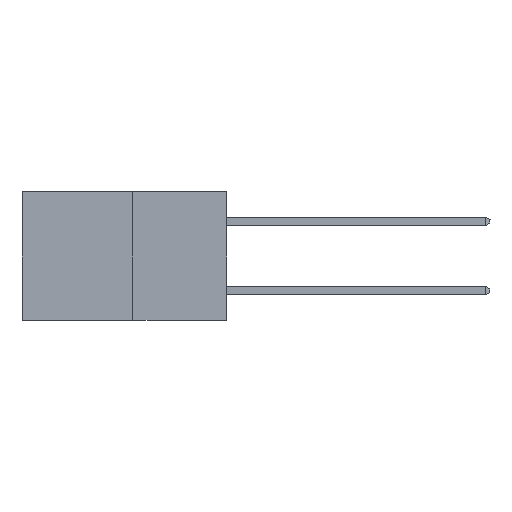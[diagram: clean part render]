
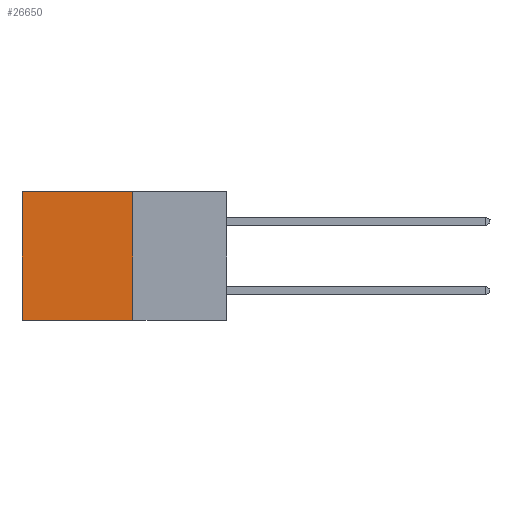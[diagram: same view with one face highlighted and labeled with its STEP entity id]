
A CAD part, left-side view. The second image highlights one B-rep face of the part: STEP entity #26650.
In plain terms, the highlighted planar face has unit normal (-1, 0, 0).
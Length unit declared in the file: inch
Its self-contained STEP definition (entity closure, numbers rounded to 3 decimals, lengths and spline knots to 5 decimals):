
#1404 = CARTESIAN_POINT ( 'NONE',  ( 0.277, 0.27, -0.37 ) ) ;
#2034 = LINE ( 'NONE', #11757, #30102 ) ;
#2102 = LINE ( 'NONE', #32947, #27060 ) ;
#2589 = CARTESIAN_POINT ( 'NONE',  ( 0.277, 0.59, 0. ) ) ;
#3235 = VERTEX_POINT ( 'NONE', #30724 ) ;
#3621 = CARTESIAN_POINT ( 'NONE',  ( 0.277, 0.59, -0.37 ) ) ;
#4065 = DIRECTION ( 'NONE',  ( 1., 0., 0. ) ) ;
#5108 = EDGE_CURVE ( 'NONE', #29380, #3235, #18339, .T. ) ;
#5743 = CARTESIAN_POINT ( 'NONE',  ( 0.277, 0.27, -0.37 ) ) ;
#5792 = DIRECTION ( 'NONE',  ( 0., 0., -1. ) ) ;
#6982 = EDGE_CURVE ( 'NONE', #18770, #32839, #2034, .T. ) ;
#7533 = VECTOR ( 'NONE', #29878, 39.37008 ) ;
#7955 = EDGE_LOOP ( 'NONE', ( #28586, #11319, #18365, #10994 ) ) ;
#9662 = DIRECTION ( 'NONE',  ( 0., 0., -1. ) ) ;
#10994 = ORIENTED_EDGE ( 'NONE', *, *, #12535, .T. ) ;
#11319 = ORIENTED_EDGE ( 'NONE', *, *, #11632, .F. ) ;
#11632 = EDGE_CURVE ( 'NONE', #3235, #32839, #21227, .T. ) ;
#11757 = CARTESIAN_POINT ( 'NONE',  ( 0.277, 0.59, -0.37 ) ) ;
#12535 = EDGE_CURVE ( 'NONE', #29380, #18770, #2102, .T. ) ;
#13899 = FACE_OUTER_BOUND ( 'NONE', #7955, .T. ) ;
#15368 = AXIS2_PLACEMENT_3D ( 'NONE', #1404, #4065, #22127 ) ;
#17039 = PLANE ( 'NONE',  #15368 ) ;
#18339 = LINE ( 'NONE', #5743, #30833 ) ;
#18365 = ORIENTED_EDGE ( 'NONE', *, *, #5108, .F. ) ;
#18770 = VERTEX_POINT ( 'NONE', #2589 ) ;
#19831 = CARTESIAN_POINT ( 'NONE',  ( 0.277, 0.27, -0.37 ) ) ;
#21227 = LINE ( 'NONE', #19831, #7533 ) ;
#22127 = DIRECTION ( 'NONE',  ( 0., 0., -1. ) ) ;
#25195 = CARTESIAN_POINT ( 'NONE',  ( 0.277, 0.27, 0. ) ) ;
#25545 = DIRECTION ( 'NONE',  ( 0., 1., 0. ) ) ;
#26650 = ADVANCED_FACE ( 'NONE', ( #13899 ), #17039, .F. ) ;
#27060 = VECTOR ( 'NONE', #25545, 39.37008 ) ;
#28586 = ORIENTED_EDGE ( 'NONE', *, *, #6982, .T. ) ;
#29380 = VERTEX_POINT ( 'NONE', #25195 ) ;
#29878 = DIRECTION ( 'NONE',  ( 0., 1., 0. ) ) ;
#30102 = VECTOR ( 'NONE', #9662, 39.37008 ) ;
#30724 = CARTESIAN_POINT ( 'NONE',  ( 0.277, 0.27, -0.37 ) ) ;
#30833 = VECTOR ( 'NONE', #5792, 39.37008 ) ;
#32839 = VERTEX_POINT ( 'NONE', #3621 ) ;
#32947 = CARTESIAN_POINT ( 'NONE',  ( 0.277, 0.27, 0. ) ) ;
